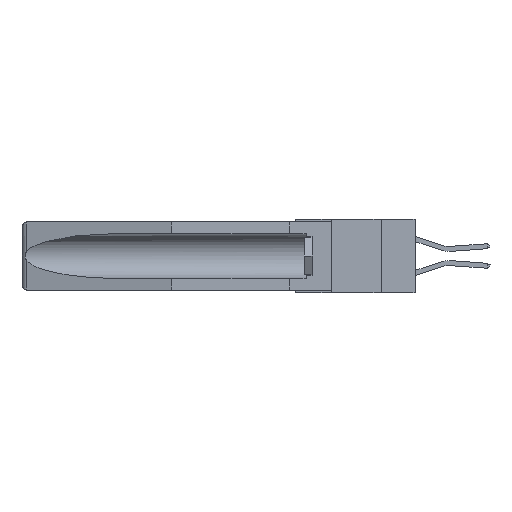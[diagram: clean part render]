
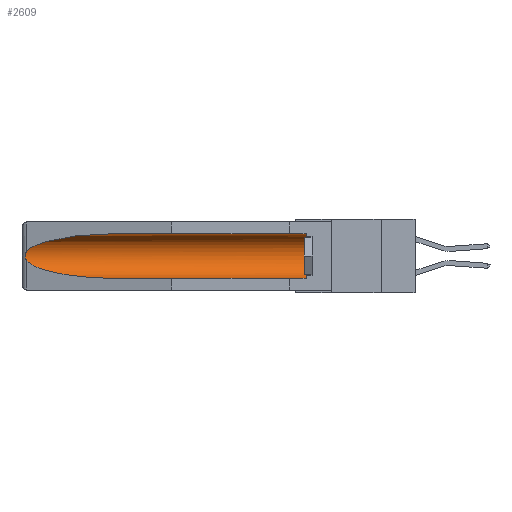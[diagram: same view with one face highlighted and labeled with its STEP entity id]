
A CAD part, left-side view. The second image highlights one B-rep face of the part: STEP entity #2609.
In plain terms, the highlighted cylindrical face has radius 2.857 mm (diameter 5.715 mm), a partial arc.
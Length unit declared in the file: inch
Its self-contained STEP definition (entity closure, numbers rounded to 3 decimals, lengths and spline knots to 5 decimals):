
#183 = CARTESIAN_POINT ( 'NONE',  ( 0.26537, 1.52718, -0.14972 ) ) ;
#271 = ORIENTED_EDGE ( 'NONE', *, *, #6742, .T. ) ;
#762 = VERTEX_POINT ( 'NONE', #3109 ) ;
#1164 = EDGE_CURVE ( 'NONE', #14772, #14689, #5411, .T. ) ;
#1268 = EDGE_CURVE ( 'NONE', #2843, #7446, #3036, .T. ) ;
#1449 = DIRECTION ( 'NONE',  ( 0., 1., 0. ) ) ;
#2130 = EDGE_CURVE ( 'NONE', #7993, #762, #4679, .T. ) ;
#2496 = CARTESIAN_POINT ( 'NONE',  ( 0.26654, 1.53092, -0.15636 ) ) ;
#2609 = ADVANCED_FACE ( 'NONE', ( #7015 ), #12545, .F. ) ;
#2670 = CARTESIAN_POINT ( 'NONE',  ( 0.25451, 1.48313, -0.24835 ) ) ;
#2697 = CARTESIAN_POINT ( 'NONE',  ( 0.26537, 1.52718, -0.14972 ) ) ;
#2843 = VERTEX_POINT ( 'NONE', #10322 ) ;
#2982 = CARTESIAN_POINT ( 'NONE',  ( 0.155, -0.30754, -0.1715 ) ) ;
#3036 = LINE ( 'NONE', #14178, #19022 ) ;
#3109 = CARTESIAN_POINT ( 'NONE',  ( 0.155, 1.07973, -0.059 ) ) ;
#3473 = ORIENTED_EDGE ( 'NONE', *, *, #7367, .T. ) ;
#3571 = AXIS2_PLACEMENT_3D ( 'NONE', #10698, #6218, #7431 ) ;
#3572 = ORIENTED_EDGE ( 'NONE', *, *, #1164, .T. ) ;
#4515 = CARTESIAN_POINT ( 'NONE',  ( 0.155, -0.30754, -0.059 ) ) ;
#4679 = LINE ( 'NONE', #4515, #7296 ) ;
#5411 = B_SPLINE_CURVE_WITH_KNOTS ( 'NONE', 3,
 ( #2697, #11650, #2496, #5679, #5601, #5463, #14642, #10159, #13382, #5736 ),
 .UNSPECIFIED., .F., .F.,
 ( 4, 2, 2, 2, 4 ),
 ( 0., 0.00029, 0.00058, 0.00087, 0.00117 ),
 .UNSPECIFIED. ) ;
#5463 = CARTESIAN_POINT ( 'NONE',  ( 0.2675, 1.53308, -0.17534 ) ) ;
#5601 = CARTESIAN_POINT ( 'NONE',  ( 0.2675, 1.53308, -0.16763 ) ) ;
#5679 = CARTESIAN_POINT ( 'NONE',  ( 0.2673, 1.5327, -0.16383 ) ) ;
#5736 = CARTESIAN_POINT ( 'NONE',  ( 0.26537, 1.52718, -0.19328 ) ) ;
#6218 = DIRECTION ( 'NONE',  ( 0., -1., 0. ) ) ;
#6742 = EDGE_CURVE ( 'NONE', #2843, #7993, #6844, .T. ) ;
#6844 = CIRCLE ( 'NONE', #3571, 0.1125 ) ;
#7015 = FACE_OUTER_BOUND ( 'NONE', #14536, .T. ) ;
#7296 = VECTOR ( 'NONE', #9124, 39.37008 ) ;
#7367 = EDGE_CURVE ( 'NONE', #762, #14772, #8747, .T. ) ;
#7431 = DIRECTION ( 'NONE',  ( 0., 0., 1. ) ) ;
#7446 = VERTEX_POINT ( 'NONE', #9607 ) ;
#7617 = CARTESIAN_POINT ( 'NONE',  ( 0.21114, 1.30732, -0.059 ) ) ;
#7993 = VERTEX_POINT ( 'NONE', #9002 ) ;
#8206 = ORIENTED_EDGE ( 'NONE', *, *, #2130, .T. ) ;
#8621 = ORIENTED_EDGE ( 'NONE', *, *, #1268, .F. ) ;
#8720 = CARTESIAN_POINT ( 'NONE',  ( 0.26537, 1.52718, -0.19328 ) ) ;
#8747 =( BOUNDED_CURVE ( )  B_SPLINE_CURVE ( 3, ( #13925, #7617, #12329, #183 ),
 .UNSPECIFIED., .F., .F. ) 
 B_SPLINE_CURVE_WITH_KNOTS ( ( 4, 4 ),
 ( 4.71239, 6.08839 ),
 .UNSPECIFIED. ) 
 CURVE ( )  GEOMETRIC_REPRESENTATION_ITEM ( )  RATIONAL_B_SPLINE_CURVE ( ( 1., 0.848, 0.848, 1. ) ) 
 REPRESENTATION_ITEM ( '' )  );
#9002 = CARTESIAN_POINT ( 'NONE',  ( 0.155, 0.126, -0.059 ) ) ;
#9124 = DIRECTION ( 'NONE',  ( 0., 1., 0. ) ) ;
#9130 = ORIENTED_EDGE ( 'NONE', *, *, #16135, .T. ) ;
#9532 = AXIS2_PLACEMENT_3D ( 'NONE', #2982, #1449, #16724 ) ;
#9607 = CARTESIAN_POINT ( 'NONE',  ( 0.155, 1.07973, -0.284 ) ) ;
#10159 = CARTESIAN_POINT ( 'NONE',  ( 0.26655, 1.53094, -0.18657 ) ) ;
#10322 = CARTESIAN_POINT ( 'NONE',  ( 0.155, 0.126, -0.284 ) ) ;
#10698 = CARTESIAN_POINT ( 'NONE',  ( 0.155, 0.126, -0.1715 ) ) ;
#11650 = CARTESIAN_POINT ( 'NONE',  ( 0.26597, 1.52961, -0.15275 ) ) ;
#11893 = CARTESIAN_POINT ( 'NONE',  ( 0.21114, 1.30732, -0.284 ) ) ;
#12329 = CARTESIAN_POINT ( 'NONE',  ( 0.25451, 1.48313, -0.09465 ) ) ;
#12545 = CYLINDRICAL_SURFACE ( 'NONE', #9532, 0.1125 ) ;
#13382 = CARTESIAN_POINT ( 'NONE',  ( 0.26597, 1.5296, -0.19026 ) ) ;
#13700 = DIRECTION ( 'NONE',  ( 0., 1., 0. ) ) ;
#13925 = CARTESIAN_POINT ( 'NONE',  ( 0.155, 1.07973, -0.059 ) ) ;
#14178 = CARTESIAN_POINT ( 'NONE',  ( 0.155, -0.30754, -0.284 ) ) ;
#14536 = EDGE_LOOP ( 'NONE', ( #3473, #3572, #9130, #8621, #271, #8206 ) ) ;
#14642 = CARTESIAN_POINT ( 'NONE',  ( 0.2673, 1.53269, -0.17917 ) ) ;
#14689 = VERTEX_POINT ( 'NONE', #8720 ) ;
#14772 = VERTEX_POINT ( 'NONE', #19596 ) ;
#14893 = CARTESIAN_POINT ( 'NONE',  ( 0.155, 1.07973, -0.284 ) ) ;
#16135 = EDGE_CURVE ( 'NONE', #14689, #7446, #19643, .T. ) ;
#16225 = CARTESIAN_POINT ( 'NONE',  ( 0.26537, 1.52718, -0.19328 ) ) ;
#16724 = DIRECTION ( 'NONE',  ( 0., 0., 1. ) ) ;
#19022 = VECTOR ( 'NONE', #13700, 39.37008 ) ;
#19596 = CARTESIAN_POINT ( 'NONE',  ( 0.26537, 1.52718, -0.14972 ) ) ;
#19643 =( BOUNDED_CURVE ( )  B_SPLINE_CURVE ( 3, ( #16225, #2670, #11893, #14893 ),
 .UNSPECIFIED., .F., .F. ) 
 B_SPLINE_CURVE_WITH_KNOTS ( ( 4, 4 ),
 ( 0.1948, 1.5708 ),
 .UNSPECIFIED. ) 
 CURVE ( )  GEOMETRIC_REPRESENTATION_ITEM ( )  RATIONAL_B_SPLINE_CURVE ( ( 1., 0.848, 0.848, 1. ) ) 
 REPRESENTATION_ITEM ( '' )  );
